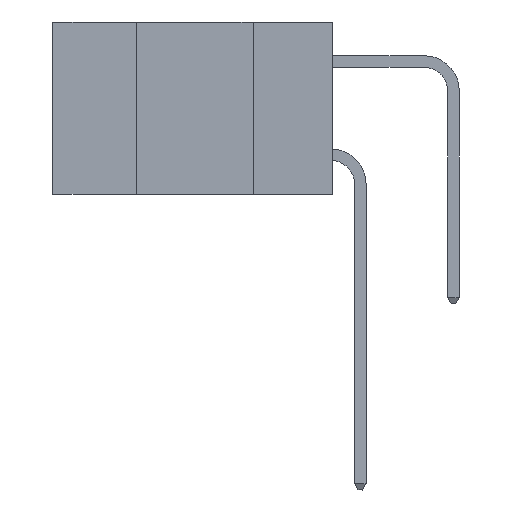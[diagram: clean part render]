
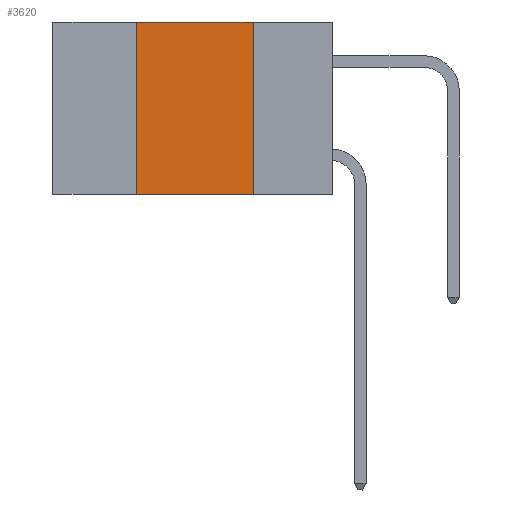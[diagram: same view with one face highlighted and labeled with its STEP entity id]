
A CAD part, left-side view. The second image highlights one B-rep face of the part: STEP entity #3620.
In plain terms, the highlighted planar face has unit normal (-1, 0, 0).
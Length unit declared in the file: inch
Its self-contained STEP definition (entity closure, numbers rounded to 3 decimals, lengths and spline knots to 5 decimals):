
#1219 = DIRECTION ( 'NONE',  ( 1., 0., 0. ) ) ;
#1241 = CARTESIAN_POINT ( 'NONE',  ( 0., 0.42, 0. ) ) ;
#1609 = DIRECTION ( 'NONE',  ( 0., 0., -1. ) ) ;
#2549 = VECTOR ( 'NONE', #1609, 39.37008 ) ;
#2580 = ORIENTED_EDGE ( 'NONE', *, *, #4948, .F. ) ;
#2732 = VECTOR ( 'NONE', #3186, 39.37008 ) ;
#2889 = LINE ( 'NONE', #8671, #2549 ) ;
#3186 = DIRECTION ( 'NONE',  ( 0., -1., 0. ) ) ;
#3541 = DIRECTION ( 'NONE',  ( 0., 0., 1. ) ) ;
#3620 = ADVANCED_FACE ( 'NONE', ( #7845 ), #10437, .F. ) ;
#3949 = CARTESIAN_POINT ( 'NONE',  ( 0., 0.17, 0. ) ) ;
#4154 = CARTESIAN_POINT ( 'NONE',  ( 0., 0.6, 0. ) ) ;
#4675 = VERTEX_POINT ( 'NONE', #5134 ) ;
#4948 = EDGE_CURVE ( 'NONE', #10005, #8177, #9245, .T. ) ;
#5109 = EDGE_CURVE ( 'NONE', #4675, #6586, #6688, .T. ) ;
#5134 = CARTESIAN_POINT ( 'NONE',  ( 0., 0.42, -0.37 ) ) ;
#5147 = AXIS2_PLACEMENT_3D ( 'NONE', #13944, #1219, #10489 ) ;
#6026 = VECTOR ( 'NONE', #3541, 39.37008 ) ;
#6470 = ORIENTED_EDGE ( 'NONE', *, *, #8607, .F. ) ;
#6586 = VERTEX_POINT ( 'NONE', #7813 ) ;
#6688 = LINE ( 'NONE', #11994, #7083 ) ;
#7083 = VECTOR ( 'NONE', #14315, 39.37008 ) ;
#7813 = CARTESIAN_POINT ( 'NONE',  ( 0., 0.17, -0.37 ) ) ;
#7845 = FACE_OUTER_BOUND ( 'NONE', #8712, .T. ) ;
#8177 = VERTEX_POINT ( 'NONE', #3949 ) ;
#8607 = EDGE_CURVE ( 'NONE', #4675, #10005, #9846, .T. ) ;
#8671 = CARTESIAN_POINT ( 'NONE',  ( 0., 0.17, 0. ) ) ;
#8712 = EDGE_LOOP ( 'NONE', ( #10237, #2580, #6470, #13448 ) ) ;
#9245 = LINE ( 'NONE', #4154, #2732 ) ;
#9846 = LINE ( 'NONE', #1241, #6026 ) ;
#10005 = VERTEX_POINT ( 'NONE', #11239 ) ;
#10237 = ORIENTED_EDGE ( 'NONE', *, *, #11633, .F. ) ;
#10437 = PLANE ( 'NONE',  #5147 ) ;
#10489 = DIRECTION ( 'NONE',  ( 0., 0., -1. ) ) ;
#11239 = CARTESIAN_POINT ( 'NONE',  ( 0., 0.42, 0. ) ) ;
#11633 = EDGE_CURVE ( 'NONE', #8177, #6586, #2889, .T. ) ;
#11994 = CARTESIAN_POINT ( 'NONE',  ( 0., 0.6, -0.37 ) ) ;
#13448 = ORIENTED_EDGE ( 'NONE', *, *, #5109, .T. ) ;
#13944 = CARTESIAN_POINT ( 'NONE',  ( 0., 0.6, 0. ) ) ;
#14315 = DIRECTION ( 'NONE',  ( 0., -1., 0. ) ) ;
